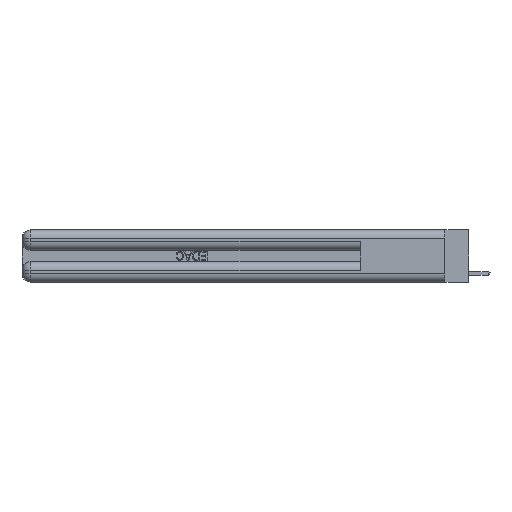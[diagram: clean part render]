
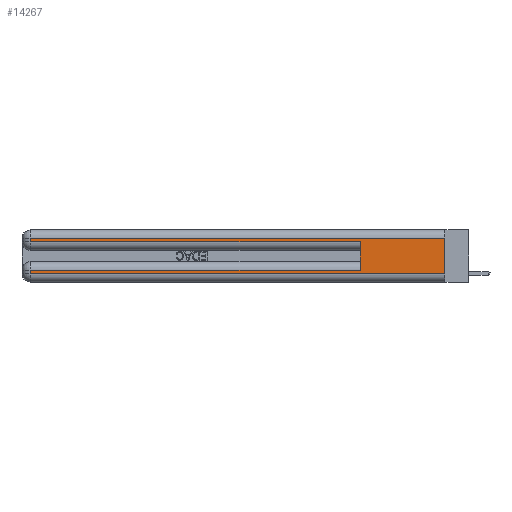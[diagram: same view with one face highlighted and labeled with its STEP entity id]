
A CAD part, left-side view. The second image highlights one B-rep face of the part: STEP entity #14267.
In plain terms, the highlighted planar face has unit normal (-1, 0, 0).
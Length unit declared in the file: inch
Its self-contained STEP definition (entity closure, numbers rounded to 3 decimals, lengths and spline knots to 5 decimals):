
#543 = LINE ( 'NONE', #29078, #15554 ) ;
#1062 = EDGE_CURVE ( 'NONE', #9097, #25413, #12108, .T. ) ;
#1340 = ORIENTED_EDGE ( 'NONE', *, *, #32543, .T. ) ;
#2687 = LINE ( 'NONE', #26529, #3488 ) ;
#3475 = DIRECTION ( 'NONE',  ( 0., 0., -1. ) ) ;
#3488 = VECTOR ( 'NONE', #8849, 39.37008 ) ;
#3515 = CARTESIAN_POINT ( 'NONE',  ( 0., 0.6, 0.285 ) ) ;
#5114 = VERTEX_POINT ( 'NONE', #27374 ) ;
#5410 = EDGE_CURVE ( 'NONE', #27092, #9097, #2687, .T. ) ;
#5519 = LINE ( 'NONE', #9098, #16625 ) ;
#5664 = DIRECTION ( 'NONE',  ( 0., -1., 0. ) ) ;
#7214 = CARTESIAN_POINT ( 'NONE',  ( 0., 0., 0.285 ) ) ;
#7476 = CARTESIAN_POINT ( 'NONE',  ( 0., 0.6, 0.085 ) ) ;
#7878 = CARTESIAN_POINT ( 'NONE',  ( 0., 0., 0.06 ) ) ;
#8307 = VERTEX_POINT ( 'NONE', #7476 ) ;
#8849 = DIRECTION ( 'NONE',  ( 0., 0., -1. ) ) ;
#8974 = CARTESIAN_POINT ( 'NONE',  ( 0., 2.94, 0.31 ) ) ;
#9097 = VERTEX_POINT ( 'NONE', #15651 ) ;
#9098 = CARTESIAN_POINT ( 'NONE',  ( 0., 0., 0.37 ) ) ;
#9313 = AXIS2_PLACEMENT_3D ( 'NONE', #27066, #19094, #31979 ) ;
#10957 = CARTESIAN_POINT ( 'NONE',  ( 0., 0., 0.31 ) ) ;
#11258 = VECTOR ( 'NONE', #13841, 39.37008 ) ;
#11540 = LINE ( 'NONE', #29193, #15892 ) ;
#11842 = EDGE_CURVE ( 'NONE', #5114, #32433, #31578, .T. ) ;
#11944 = EDGE_CURVE ( 'NONE', #8307, #32346, #26001, .T. ) ;
#12108 = LINE ( 'NONE', #7214, #13280 ) ;
#12447 = VECTOR ( 'NONE', #13508, 39.37008 ) ;
#13280 = VECTOR ( 'NONE', #27524, 39.37008 ) ;
#13508 = DIRECTION ( 'NONE',  ( 0., 1., 0. ) ) ;
#13841 = DIRECTION ( 'NONE',  ( 0., 1., 0. ) ) ;
#13896 = FACE_OUTER_BOUND ( 'NONE', #28493, .T. ) ;
#14096 = EDGE_CURVE ( 'NONE', #32346, #5114, #11540, .T. ) ;
#14267 = ADVANCED_FACE ( 'NONE', ( #13896 ), #14280, .F. ) ;
#14280 = PLANE ( 'NONE',  #9313 ) ;
#14462 = ORIENTED_EDGE ( 'NONE', *, *, #23757, .F. ) ;
#15554 = VECTOR ( 'NONE', #21756, 39.37008 ) ;
#15651 = CARTESIAN_POINT ( 'NONE',  ( 0., 2.94, 0.285 ) ) ;
#15892 = VECTOR ( 'NONE', #3475, 39.37008 ) ;
#16625 = VECTOR ( 'NONE', #24658, 39.37008 ) ;
#18916 = ORIENTED_EDGE ( 'NONE', *, *, #27641, .F. ) ;
#19094 = DIRECTION ( 'NONE',  ( 1., 0., 0. ) ) ;
#19424 = CARTESIAN_POINT ( 'NONE',  ( 0., 0., 0.31 ) ) ;
#19527 = ORIENTED_EDGE ( 'NONE', *, *, #5410, .T. ) ;
#19594 = VERTEX_POINT ( 'NONE', #19424 ) ;
#20066 = VECTOR ( 'NONE', #5664, 39.37008 ) ;
#21756 = DIRECTION ( 'NONE',  ( 0., 0., 1. ) ) ;
#22858 = ORIENTED_EDGE ( 'NONE', *, *, #14096, .T. ) ;
#23757 = EDGE_CURVE ( 'NONE', #19594, #32433, #5519, .T. ) ;
#24658 = DIRECTION ( 'NONE',  ( 0., 0., -1. ) ) ;
#25412 = CARTESIAN_POINT ( 'NONE',  ( 0., 2.94, 0.085 ) ) ;
#25413 = VERTEX_POINT ( 'NONE', #3515 ) ;
#25983 = LINE ( 'NONE', #10957, #12447 ) ;
#26001 = LINE ( 'NONE', #26421, #11258 ) ;
#26421 = CARTESIAN_POINT ( 'NONE',  ( 0., 0., 0.085 ) ) ;
#26529 = CARTESIAN_POINT ( 'NONE',  ( 0., 2.94, 0.37 ) ) ;
#27066 = CARTESIAN_POINT ( 'NONE',  ( 0., 0., 0.37 ) ) ;
#27092 = VERTEX_POINT ( 'NONE', #8974 ) ;
#27374 = CARTESIAN_POINT ( 'NONE',  ( 0., 2.94, 0.06 ) ) ;
#27524 = DIRECTION ( 'NONE',  ( 0., -1., 0. ) ) ;
#27641 = EDGE_CURVE ( 'NONE', #8307, #25413, #543, .T. ) ;
#28489 = ORIENTED_EDGE ( 'NONE', *, *, #1062, .T. ) ;
#28493 = EDGE_LOOP ( 'NONE', ( #14462, #1340, #19527, #28489, #18916, #32319, #22858, #32596 ) ) ;
#29078 = CARTESIAN_POINT ( 'NONE',  ( 0., 0.6, 0.145 ) ) ;
#29193 = CARTESIAN_POINT ( 'NONE',  ( 0., 2.94, 0.37 ) ) ;
#31448 = CARTESIAN_POINT ( 'NONE',  ( 0., 0., 0.06 ) ) ;
#31578 = LINE ( 'NONE', #31448, #20066 ) ;
#31979 = DIRECTION ( 'NONE',  ( 0., 0., -1. ) ) ;
#32319 = ORIENTED_EDGE ( 'NONE', *, *, #11944, .T. ) ;
#32346 = VERTEX_POINT ( 'NONE', #25412 ) ;
#32433 = VERTEX_POINT ( 'NONE', #7878 ) ;
#32543 = EDGE_CURVE ( 'NONE', #19594, #27092, #25983, .T. ) ;
#32596 = ORIENTED_EDGE ( 'NONE', *, *, #11842, .T. ) ;
